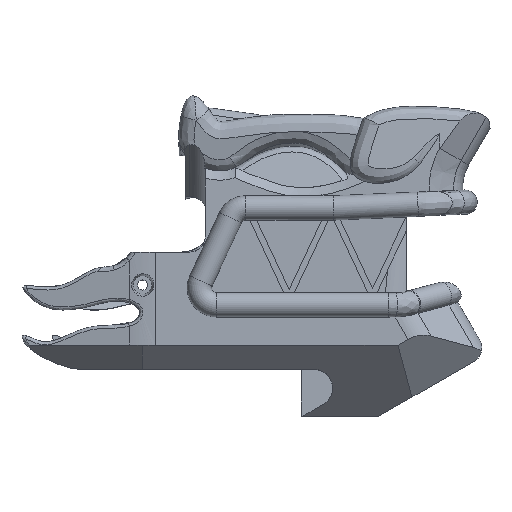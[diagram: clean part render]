
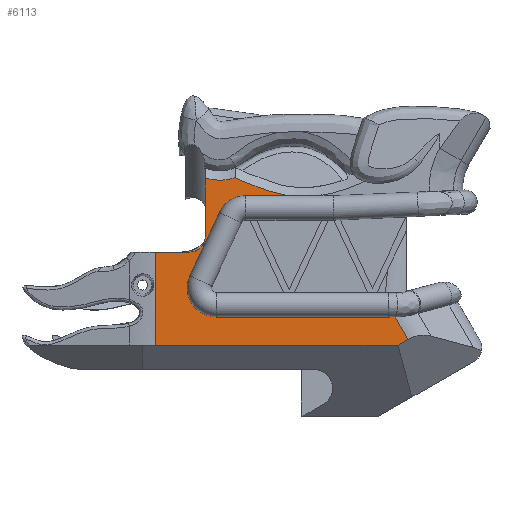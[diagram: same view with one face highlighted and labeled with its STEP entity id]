
A CAD part, left-side view. The second image highlights one B-rep face of the part: STEP entity #6113.
In plain terms, the highlighted planar face has unit normal (-1, 0, 0).
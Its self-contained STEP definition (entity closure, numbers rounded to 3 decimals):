
#117=CIRCLE('',#6302,9.5);
#140=CIRCLE('',#6363,5.);
#180=CIRCLE('',#6502,9.5);
#484=B_SPLINE_CURVE_WITH_KNOTS('',3,(#12230,#12231,#12232,#12233,#12234,
#12235),.UNSPECIFIED.,.F.,.F.,(4,2,4),(0.,0.103,
0.201),.UNSPECIFIED.);
#518=B_SPLINE_CURVE_WITH_KNOTS('',3,(#13729,#13730,#13731,#13732,#13733,
#13734,#13735,#13736,#13737,#13738),.UNSPECIFIED.,.F.,.F.,(4,1,1,1,1,1,
1,4),(-7.477,-7.198,-7.057,-6.915,
-6.632,-6.348,-5.782,-5.308),
 .UNSPECIFIED.);
#531=B_SPLINE_CURVE_WITH_KNOTS('',3,(#13865,#13866,#13867,#13868,#13869),
 .UNSPECIFIED.,.F.,.F.,(4,1,4),(-7.892,-7.481,-7.477),
 .UNSPECIFIED.);
#533=B_SPLINE_CURVE_WITH_KNOTS('',3,(#13906,#13907,#13908,#13909,#13910,
#13911,#13912,#13913),.UNSPECIFIED.,.F.,.F.,(4,2,2,4),(-1.009,
-0.606,-0.182,0.),.UNSPECIFIED.);
#1075=FACE_OUTER_BOUND('',#1378,.T.);
#1378=EDGE_LOOP('',(#5603,#5604,#5605,#5606,#5607,#5608,#5609,#5610,#5611,
#5612,#5613,#5614,#5615,#5616,#5617,#5618));
#1437=LINE('',#8306,#1793);
#1466=LINE('',#8403,#1822);
#1511=LINE('',#9158,#1867);
#1601=LINE('',#11521,#1957);
#1602=LINE('',#12146,#1958);
#1654=LINE('',#13615,#2010);
#1655=LINE('',#13618,#2011);
#1741=LINE('',#28772,#2097);
#1742=LINE('',#28777,#2098);
#1793=VECTOR('',#6600,10.);
#1822=VECTOR('',#6677,10.);
#1867=VECTOR('',#6770,10.);
#1957=VECTOR('',#7074,10.);
#1958=VECTOR('',#7091,10.);
#2010=VECTOR('',#7255,10.);
#2011=VECTOR('',#7258,10.);
#2097=VECTOR('',#7620,10.);
#2098=VECTOR('',#7629,10.);
#2154=VERTEX_POINT('',#8303);
#2155=VERTEX_POINT('',#8305);
#2187=VERTEX_POINT('',#8401);
#2230=VERTEX_POINT('',#9156);
#2380=VERTEX_POINT('',#11520);
#2390=VERTEX_POINT('',#12135);
#2392=VERTEX_POINT('',#12139);
#2394=VERTEX_POINT('',#12145);
#2470=VERTEX_POINT('',#13613);
#2471=VERTEX_POINT('',#13617);
#2473=VERTEX_POINT('',#13623);
#2478=VERTEX_POINT('',#13727);
#2479=VERTEX_POINT('',#13728);
#2491=VERTEX_POINT('',#13858);
#2492=VERTEX_POINT('',#13898);
#2772=VERTEX_POINT('',#28771);
#2842=EDGE_CURVE('',#2154,#2155,#1437,.T.);
#2886=EDGE_CURVE('',#2187,#2154,#1466,.T.);
#2950=EDGE_CURVE('',#2230,#2187,#1511,.T.);
#3165=EDGE_CURVE('',#2155,#2380,#1601,.T.);
#3182=EDGE_CURVE('',#2390,#2392,#117,.T.);
#3184=EDGE_CURVE('',#2394,#2390,#1602,.T.);
#3188=EDGE_CURVE('',#2230,#2394,#484,.T.);
#3300=EDGE_CURVE('',#2392,#2470,#1654,.T.);
#3301=EDGE_CURVE('',#2380,#2471,#1655,.T.);
#3304=EDGE_CURVE('',#2471,#2473,#140,.T.);
#3315=EDGE_CURVE('',#2478,#2479,#518,.T.);
#3328=EDGE_CURVE('',#2491,#2478,#531,.T.);
#3330=EDGE_CURVE('',#2492,#2491,#533,.F.);
#3733=EDGE_CURVE('',#2772,#2479,#1741,.T.);
#3735=EDGE_CURVE('',#2470,#2772,#180,.T.);
#3736=EDGE_CURVE('',#2473,#2492,#1742,.T.);
#5603=ORIENTED_EDGE('',*,*,#3735,.T.);
#5604=ORIENTED_EDGE('',*,*,#3733,.T.);
#5605=ORIENTED_EDGE('',*,*,#3315,.F.);
#5606=ORIENTED_EDGE('',*,*,#3328,.F.);
#5607=ORIENTED_EDGE('',*,*,#3330,.F.);
#5608=ORIENTED_EDGE('',*,*,#3736,.F.);
#5609=ORIENTED_EDGE('',*,*,#3304,.F.);
#5610=ORIENTED_EDGE('',*,*,#3301,.F.);
#5611=ORIENTED_EDGE('',*,*,#3165,.F.);
#5612=ORIENTED_EDGE('',*,*,#2842,.F.);
#5613=ORIENTED_EDGE('',*,*,#2886,.F.);
#5614=ORIENTED_EDGE('',*,*,#2950,.F.);
#5615=ORIENTED_EDGE('',*,*,#3188,.T.);
#5616=ORIENTED_EDGE('',*,*,#3184,.T.);
#5617=ORIENTED_EDGE('',*,*,#3182,.T.);
#5618=ORIENTED_EDGE('',*,*,#3300,.T.);
#5824=PLANE('',#6503);
#6113=ADVANCED_FACE('',(#1075),#5824,.T.);
#6302=AXIS2_PLACEMENT_3D('',#12141,#7085,#7086);
#6363=AXIS2_PLACEMENT_3D('',#13624,#7263,#7264);
#6502=AXIS2_PLACEMENT_3D('',#28775,#7625,#7626);
#6503=AXIS2_PLACEMENT_3D('',#28776,#7627,#7628);
#6600=DIRECTION('',(0.,1.,0.));
#6677=DIRECTION('',(0.,0.866,-0.5));
#6770=DIRECTION('',(0.,-0.5,-0.866));
#7074=DIRECTION('',(0.,0.,1.));
#7085=DIRECTION('center_axis',(1.,0.,0.));
#7086=DIRECTION('ref_axis',(0.,0.,1.));
#7091=DIRECTION('',(0.,1.,0.));
#7255=DIRECTION('',(0.,-0.423,0.906));
#7258=DIRECTION('',(0.,-1.,0.));
#7263=DIRECTION('center_axis',(-1.,0.,0.));
#7264=DIRECTION('ref_axis',(0.,-1.,0.));
#7620=DIRECTION('',(0.,-1.,0.));
#7625=DIRECTION('center_axis',(1.,0.,0.));
#7626=DIRECTION('ref_axis',(0.,0.,1.));
#7627=DIRECTION('center_axis',(-1.,0.,0.));
#7628=DIRECTION('ref_axis',(0.,-1.,0.));
#7629=DIRECTION('',(0.,0.,1.));
#8303=CARTESIAN_POINT('',(-30.,-46.618,-42.08));
#8305=CARTESIAN_POINT('',(-30.,32.796,-42.08));
#8306=CARTESIAN_POINT('',(-30.,-37.98,-42.08));
#8401=CARTESIAN_POINT('',(-30.,-49.925,-40.171));
#8403=CARTESIAN_POINT('',(-30.,-3.294,-67.093));
#9156=CARTESIAN_POINT('',(-30.,-45.712,-32.873));
#9158=CARTESIAN_POINT('',(-30.,1.616,49.1));
#11520=CARTESIAN_POINT('',(-30.,32.796,-11.571));
#11521=CARTESIAN_POINT('',(-30.,32.796,26.798));
#12135=CARTESIAN_POINT('',(-30.,13.004,-32.878));
#12139=CARTESIAN_POINT('',(-30.,21.614,-19.363));
#12141=CARTESIAN_POINT('Origin',(-30.,13.004,-23.378));
#12145=CARTESIAN_POINT('',(-30.,-43.405,-32.878));
#12146=CARTESIAN_POINT('',(-30.,53.004,-32.878));
#12230=CARTESIAN_POINT('Ctrl Pts',(-30.,-45.712,-32.873));
#12231=CARTESIAN_POINT('Ctrl Pts',(-30.,-45.369,-32.876));
#12232=CARTESIAN_POINT('Ctrl Pts',(-30.,-45.008,
-32.877));
#12233=CARTESIAN_POINT('Ctrl Pts',(-30.,-44.356,
-32.878));
#12234=CARTESIAN_POINT('Ctrl Pts',(-30.,-43.999,-32.878));
#12235=CARTESIAN_POINT('Ctrl Pts',(-30.,-43.405,-32.878));
#13613=CARTESIAN_POINT('',(-30.,11.938,1.388));
#13615=CARTESIAN_POINT('',(-30.,11.938,1.388));
#13617=CARTESIAN_POINT('',(-30.,21.611,-11.571));
#13618=CARTESIAN_POINT('',(-30.,41.253,-11.571));
#13623=CARTESIAN_POINT('',(-30.,16.611,-6.571));
#13624=CARTESIAN_POINT('Origin',(-30.,21.611,-6.571));
#13727=CARTESIAN_POINT('',(-30.,3.905,11.515));
#13728=CARTESIAN_POINT('',(-30.,-10.814,6.873));
#13729=CARTESIAN_POINT('Ctrl Pts',(-30.,3.905,11.515));
#13730=CARTESIAN_POINT('Ctrl Pts',(-30.,3.299,11.248));
#13731=CARTESIAN_POINT('Ctrl Pts',(-30.,2.401,10.861));
#13732=CARTESIAN_POINT('Ctrl Pts',(-30.,1.147,10.345));
#13733=CARTESIAN_POINT('Ctrl Pts',(-30.,-0.222,9.8));
#13734=CARTESIAN_POINT('Ctrl Pts',(-30.,-2.012,9.131));
#13735=CARTESIAN_POINT('Ctrl Pts',(-30.,-4.678,8.233));
#13736=CARTESIAN_POINT('Ctrl Pts',(-30.,-7.633,7.418));
#13737=CARTESIAN_POINT('Ctrl Pts',(-30.,-9.831,7.012));
#13738=CARTESIAN_POINT('Ctrl Pts',(-30.,-10.814,6.873));
#13858=CARTESIAN_POINT('',(-30.,6.79,12.837));
#13865=CARTESIAN_POINT('Ctrl Pts',(-30.,6.789,12.836));
#13866=CARTESIAN_POINT('Ctrl Pts',(-30.,5.748,12.34));
#13867=CARTESIAN_POINT('Ctrl Pts',(-30.,4.819,11.918));
#13868=CARTESIAN_POINT('Ctrl Pts',(-30.,3.915,11.519));
#13869=CARTESIAN_POINT('Ctrl Pts',(-30.,3.905,11.515));
#13898=CARTESIAN_POINT('',(-30.,16.611,12.728));
#13906=CARTESIAN_POINT('Ctrl Pts',(-30.,6.79,12.837));
#13907=CARTESIAN_POINT('Ctrl Pts',(-30.,8.041,12.376));
#13908=CARTESIAN_POINT('Ctrl Pts',(-30.,9.302,12.105));
#13909=CARTESIAN_POINT('Ctrl Pts',(-30.,12.035,11.924));
#13910=CARTESIAN_POINT('Ctrl Pts',(-30.,13.455,12.035));
#13911=CARTESIAN_POINT('Ctrl Pts',(-30.,15.439,12.417));
#13912=CARTESIAN_POINT('Ctrl Pts',(-30.,16.03,12.56));
#13913=CARTESIAN_POINT('Ctrl Pts',(-30.,16.611,12.728));
#28771=CARTESIAN_POINT('',(-30.,3.328,6.873));
#28772=CARTESIAN_POINT('',(-30.,-65.318,6.873));
#28775=CARTESIAN_POINT('Origin',(-30.,3.328,-2.627));
#28776=CARTESIAN_POINT('Origin',(-30.,37.17,26.798));
#28777=CARTESIAN_POINT('',(-30.,16.611,5.999));
